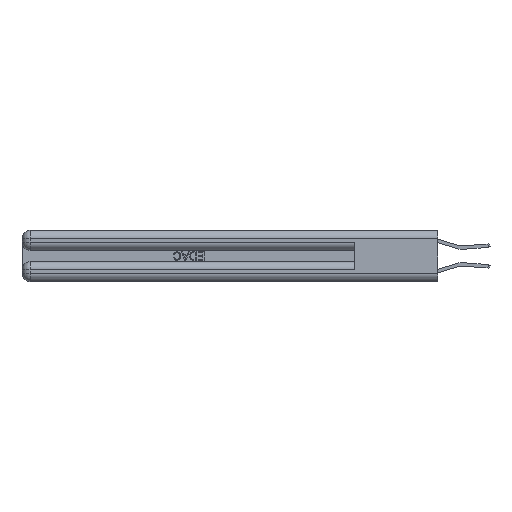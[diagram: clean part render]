
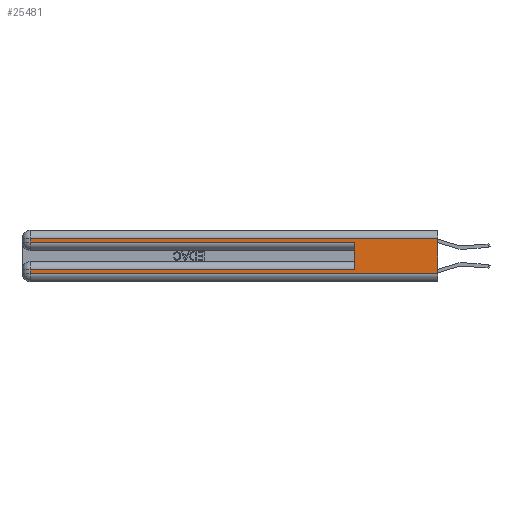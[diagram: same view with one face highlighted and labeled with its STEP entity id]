
A CAD part, left-side view. The second image highlights one B-rep face of the part: STEP entity #25481.
In plain terms, the highlighted planar face has unit normal (-1, 0, 0).
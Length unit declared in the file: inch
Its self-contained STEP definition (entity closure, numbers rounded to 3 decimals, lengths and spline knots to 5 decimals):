
#426 = LINE ( 'NONE', #28024, #13391 ) ;
#509 = ORIENTED_EDGE ( 'NONE', *, *, #30105, .T. ) ;
#653 = AXIS2_PLACEMENT_3D ( 'NONE', #31728, #6632, #12404 ) ;
#1337 = CARTESIAN_POINT ( 'NONE',  ( 0., 2.94, 0.37 ) ) ;
#2894 = DIRECTION ( 'NONE',  ( 0., 0., 1. ) ) ;
#3528 = LINE ( 'NONE', #31283, #23890 ) ;
#3708 = CARTESIAN_POINT ( 'NONE',  ( 0., 0., 0.37 ) ) ;
#3802 = DIRECTION ( 'NONE',  ( 0., 0., -1. ) ) ;
#4154 = EDGE_CURVE ( 'NONE', #16009, #6543, #16122, .T. ) ;
#5539 = LINE ( 'NONE', #26967, #32292 ) ;
#6285 = LINE ( 'NONE', #1337, #18495 ) ;
#6543 = VERTEX_POINT ( 'NONE', #14111 ) ;
#6632 = DIRECTION ( 'NONE',  ( 1., 0., 0. ) ) ;
#10052 = DIRECTION ( 'NONE',  ( 0., 0., -1. ) ) ;
#10295 = CARTESIAN_POINT ( 'NONE',  ( 0., 0., 0.06 ) ) ;
#10850 = DIRECTION ( 'NONE',  ( 0., 0., -1. ) ) ;
#11169 = VERTEX_POINT ( 'NONE', #11480 ) ;
#11480 = CARTESIAN_POINT ( 'NONE',  ( 0., 2.94, 0.285 ) ) ;
#12404 = DIRECTION ( 'NONE',  ( 0., 0., -1. ) ) ;
#12811 = CARTESIAN_POINT ( 'NONE',  ( 0., 0.6, 0.145 ) ) ;
#13391 = VECTOR ( 'NONE', #23055, 39.37008 ) ;
#13421 = CARTESIAN_POINT ( 'NONE',  ( 0., 2.94, 0.31 ) ) ;
#14049 = VERTEX_POINT ( 'NONE', #17950 ) ;
#14111 = CARTESIAN_POINT ( 'NONE',  ( 0., 0., 0.06 ) ) ;
#14462 = VERTEX_POINT ( 'NONE', #28944 ) ;
#14494 = CARTESIAN_POINT ( 'NONE',  ( 0., 2.94, 0.37 ) ) ;
#14795 = VECTOR ( 'NONE', #25170, 39.37008 ) ;
#16009 = VERTEX_POINT ( 'NONE', #21548 ) ;
#16122 = LINE ( 'NONE', #3708, #31138 ) ;
#17534 = VERTEX_POINT ( 'NONE', #13421 ) ;
#17950 = CARTESIAN_POINT ( 'NONE',  ( 0., 2.94, 0.085 ) ) ;
#18495 = VECTOR ( 'NONE', #3802, 39.37008 ) ;
#18549 = VERTEX_POINT ( 'NONE', #27398 ) ;
#19014 = ORIENTED_EDGE ( 'NONE', *, *, #25283, .F. ) ;
#19480 = ORIENTED_EDGE ( 'NONE', *, *, #4154, .F. ) ;
#20521 = LINE ( 'NONE', #10295, #14795 ) ;
#20733 = LINE ( 'NONE', #12811, #27554 ) ;
#21039 = DIRECTION ( 'NONE',  ( 0., -1., 0. ) ) ;
#21068 = ORIENTED_EDGE ( 'NONE', *, *, #23754, .T. ) ;
#21548 = CARTESIAN_POINT ( 'NONE',  ( 0., 0., 0.31 ) ) ;
#21656 = PLANE ( 'NONE',  #653 ) ;
#22650 = ORIENTED_EDGE ( 'NONE', *, *, #28922, .T. ) ;
#22676 = ORIENTED_EDGE ( 'NONE', *, *, #27067, .T. ) ;
#22884 = VERTEX_POINT ( 'NONE', #31715 ) ;
#23055 = DIRECTION ( 'NONE',  ( 0., 1., 0. ) ) ;
#23754 = EDGE_CURVE ( 'NONE', #22884, #6543, #20521, .T. ) ;
#23780 = EDGE_CURVE ( 'NONE', #17534, #11169, #6285, .T. ) ;
#23890 = VECTOR ( 'NONE', #21039, 39.37008 ) ;
#25153 = ORIENTED_EDGE ( 'NONE', *, *, #25328, .T. ) ;
#25170 = DIRECTION ( 'NONE',  ( 0., -1., 0. ) ) ;
#25270 = ORIENTED_EDGE ( 'NONE', *, *, #23780, .T. ) ;
#25283 = EDGE_CURVE ( 'NONE', #14462, #18549, #20733, .T. ) ;
#25328 = EDGE_CURVE ( 'NONE', #14462, #14049, #5539, .T. ) ;
#25477 = VECTOR ( 'NONE', #10052, 39.37008 ) ;
#25481 = ADVANCED_FACE ( 'NONE', ( #29441 ), #21656, .F. ) ;
#26967 = CARTESIAN_POINT ( 'NONE',  ( 0., 0., 0.085 ) ) ;
#27067 = EDGE_CURVE ( 'NONE', #14049, #22884, #30206, .T. ) ;
#27133 = DIRECTION ( 'NONE',  ( 0., 1., 0. ) ) ;
#27398 = CARTESIAN_POINT ( 'NONE',  ( 0., 0.6, 0.285 ) ) ;
#27554 = VECTOR ( 'NONE', #2894, 39.37008 ) ;
#28024 = CARTESIAN_POINT ( 'NONE',  ( 0., 0., 0.31 ) ) ;
#28922 = EDGE_CURVE ( 'NONE', #16009, #17534, #426, .T. ) ;
#28944 = CARTESIAN_POINT ( 'NONE',  ( 0., 0.6, 0.085 ) ) ;
#29231 = EDGE_LOOP ( 'NONE', ( #19480, #22650, #25270, #509, #19014, #25153, #22676, #21068 ) ) ;
#29441 = FACE_OUTER_BOUND ( 'NONE', #29231, .T. ) ;
#30105 = EDGE_CURVE ( 'NONE', #11169, #18549, #3528, .T. ) ;
#30206 = LINE ( 'NONE', #14494, #25477 ) ;
#31138 = VECTOR ( 'NONE', #10850, 39.37008 ) ;
#31283 = CARTESIAN_POINT ( 'NONE',  ( 0., 0., 0.285 ) ) ;
#31715 = CARTESIAN_POINT ( 'NONE',  ( 0., 2.94, 0.06 ) ) ;
#31728 = CARTESIAN_POINT ( 'NONE',  ( 0., 0., 0.37 ) ) ;
#32292 = VECTOR ( 'NONE', #27133, 39.37008 ) ;
